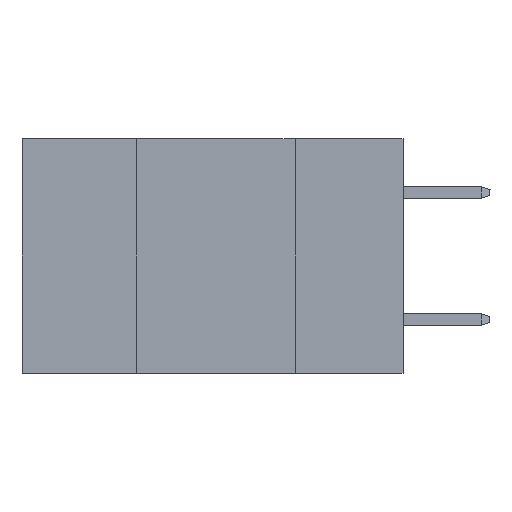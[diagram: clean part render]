
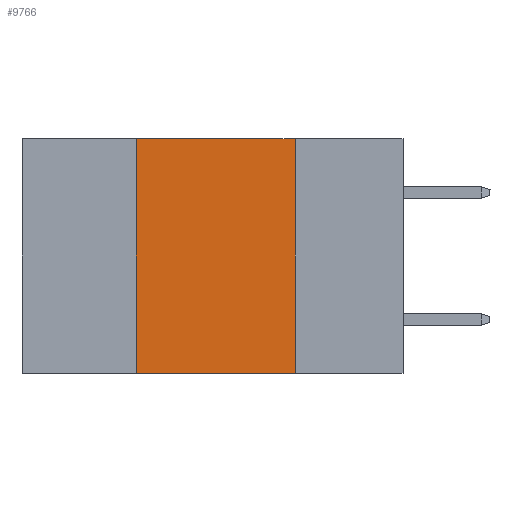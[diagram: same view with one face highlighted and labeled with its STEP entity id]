
A CAD part, left-side view. The second image highlights one B-rep face of the part: STEP entity #9766.
In plain terms, the highlighted planar face has unit normal (-1, 0, 0).
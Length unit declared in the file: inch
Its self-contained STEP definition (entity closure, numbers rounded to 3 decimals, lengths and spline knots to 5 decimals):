
#812 = ORIENTED_EDGE ( 'NONE', *, *, #8616, .F. ) ;
#873 = VERTEX_POINT ( 'NONE', #17637 ) ;
#1264 = CARTESIAN_POINT ( 'NONE',  ( 0., 0.42, -0.37 ) ) ;
#1805 = DIRECTION ( 'NONE',  ( 0., 0., 1. ) ) ;
#2060 = CARTESIAN_POINT ( 'NONE',  ( 0., 0.42, 0. ) ) ;
#2189 = CARTESIAN_POINT ( 'NONE',  ( 0., 0.17, -0.37 ) ) ;
#2288 = VERTEX_POINT ( 'NONE', #2189 ) ;
#3302 = DIRECTION ( 'NONE',  ( 0., -1., 0. ) ) ;
#3489 = CARTESIAN_POINT ( 'NONE',  ( 0., 0.6, 0. ) ) ;
#3700 = AXIS2_PLACEMENT_3D ( 'NONE', #7448, #6296, #16559 ) ;
#4224 = EDGE_LOOP ( 'NONE', ( #16972, #11178, #812, #15757 ) ) ;
#5712 = EDGE_CURVE ( 'NONE', #10431, #2288, #7316, .T. ) ;
#6212 = FACE_OUTER_BOUND ( 'NONE', #4224, .T. ) ;
#6296 = DIRECTION ( 'NONE',  ( 1., 0., 0. ) ) ;
#6858 = VERTEX_POINT ( 'NONE', #2060 ) ;
#7313 = CARTESIAN_POINT ( 'NONE',  ( 0., 0.42, 0. ) ) ;
#7316 = LINE ( 'NONE', #14418, #14896 ) ;
#7448 = CARTESIAN_POINT ( 'NONE',  ( 0., 0.6, 0. ) ) ;
#7733 = PLANE ( 'NONE',  #3700 ) ;
#7763 = LINE ( 'NONE', #9385, #13966 ) ;
#8616 = EDGE_CURVE ( 'NONE', #10431, #6858, #9039, .T. ) ;
#9039 = LINE ( 'NONE', #7313, #14941 ) ;
#9198 = LINE ( 'NONE', #3489, #10601 ) ;
#9385 = CARTESIAN_POINT ( 'NONE',  ( 0., 0.17, 0. ) ) ;
#9766 = ADVANCED_FACE ( 'NONE', ( #6212 ), #7733, .F. ) ;
#10431 = VERTEX_POINT ( 'NONE', #1264 ) ;
#10601 = VECTOR ( 'NONE', #3302, 39.37008 ) ;
#11134 = EDGE_CURVE ( 'NONE', #873, #2288, #7763, .T. ) ;
#11153 = EDGE_CURVE ( 'NONE', #6858, #873, #9198, .T. ) ;
#11178 = ORIENTED_EDGE ( 'NONE', *, *, #11153, .F. ) ;
#13186 = DIRECTION ( 'NONE',  ( 0., -1., 0. ) ) ;
#13785 = DIRECTION ( 'NONE',  ( 0., 0., -1. ) ) ;
#13966 = VECTOR ( 'NONE', #13785, 39.37008 ) ;
#14418 = CARTESIAN_POINT ( 'NONE',  ( 0., 0.6, -0.37 ) ) ;
#14896 = VECTOR ( 'NONE', #13186, 39.37008 ) ;
#14941 = VECTOR ( 'NONE', #1805, 39.37008 ) ;
#15757 = ORIENTED_EDGE ( 'NONE', *, *, #5712, .T. ) ;
#16559 = DIRECTION ( 'NONE',  ( 0., 0., -1. ) ) ;
#16972 = ORIENTED_EDGE ( 'NONE', *, *, #11134, .F. ) ;
#17637 = CARTESIAN_POINT ( 'NONE',  ( 0., 0.17, 0. ) ) ;
